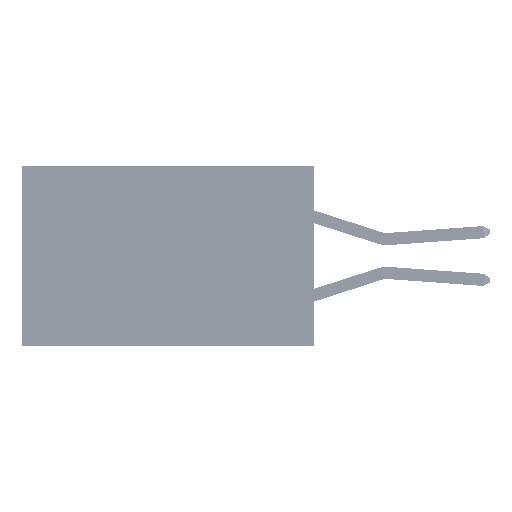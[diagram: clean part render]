
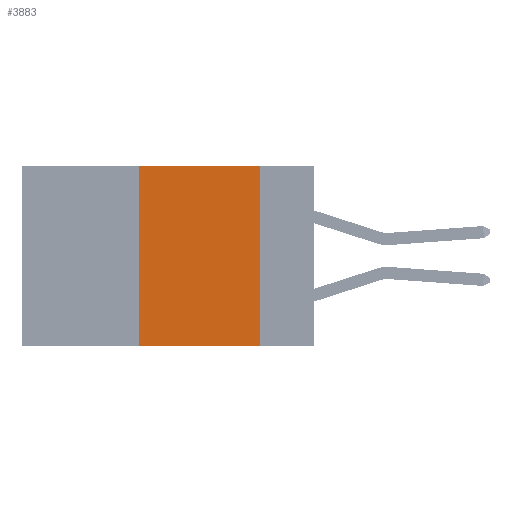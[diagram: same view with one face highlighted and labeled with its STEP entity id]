
A CAD part, left-side view. The second image highlights one B-rep face of the part: STEP entity #3883.
In plain terms, the highlighted planar face has unit normal (-1, 0, 0).
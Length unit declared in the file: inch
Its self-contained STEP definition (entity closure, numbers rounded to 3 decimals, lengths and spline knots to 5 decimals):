
#3260 = VERTEX_POINT ( 'NONE', #17033 ) ;
#3572 = AXIS2_PLACEMENT_3D ( 'NONE', #42598, #31420, #8607 ) ;
#3883 = ADVANCED_FACE ( 'NONE', ( #20816 ), #23751, .F. ) ;
#4056 = LINE ( 'NONE', #18762, #48701 ) ;
#6908 = DIRECTION ( 'NONE',  ( 0., -1., 0. ) ) ;
#8607 = DIRECTION ( 'NONE',  ( 0., 0., -1. ) ) ;
#8686 = DIRECTION ( 'NONE',  ( 0., 0., -1. ) ) ;
#10719 = EDGE_LOOP ( 'NONE', ( #48430, #15231, #14792, #28986 ) ) ;
#12511 = CARTESIAN_POINT ( 'NONE',  ( 0., 0.11, 0. ) ) ;
#13696 = CARTESIAN_POINT ( 'NONE',  ( 0., 0.11, -0.37 ) ) ;
#14792 = ORIENTED_EDGE ( 'NONE', *, *, #29529, .F. ) ;
#15231 = ORIENTED_EDGE ( 'NONE', *, *, #34833, .F. ) ;
#17016 = LINE ( 'NONE', #45388, #19379 ) ;
#17033 = CARTESIAN_POINT ( 'NONE',  ( 0., 0.11, 0. ) ) ;
#17497 = CARTESIAN_POINT ( 'NONE',  ( 0., 0.36, -0.37 ) ) ;
#18762 = CARTESIAN_POINT ( 'NONE',  ( 0., 0.6, 0. ) ) ;
#19090 = VECTOR ( 'NONE', #42324, 39.37008 ) ;
#19379 = VECTOR ( 'NONE', #46019, 39.37008 ) ;
#20316 = VERTEX_POINT ( 'NONE', #17497 ) ;
#20816 = FACE_OUTER_BOUND ( 'NONE', #10719, .T. ) ;
#21238 = CARTESIAN_POINT ( 'NONE',  ( 0., 0.36, 0. ) ) ;
#23751 = PLANE ( 'NONE',  #3572 ) ;
#25722 = VECTOR ( 'NONE', #8686, 39.37008 ) ;
#28986 = ORIENTED_EDGE ( 'NONE', *, *, #46115, .T. ) ;
#29529 = EDGE_CURVE ( 'NONE', #20316, #42090, #34529, .T. ) ;
#31420 = DIRECTION ( 'NONE',  ( 1., 0., 0. ) ) ;
#34529 = LINE ( 'NONE', #42477, #19090 ) ;
#34833 = EDGE_CURVE ( 'NONE', #42090, #3260, #4056, .T. ) ;
#40669 = EDGE_CURVE ( 'NONE', #3260, #48290, #45989, .T. ) ;
#42090 = VERTEX_POINT ( 'NONE', #21238 ) ;
#42324 = DIRECTION ( 'NONE',  ( 0., 0., 1. ) ) ;
#42477 = CARTESIAN_POINT ( 'NONE',  ( 0., 0.36, 0. ) ) ;
#42598 = CARTESIAN_POINT ( 'NONE',  ( 0., 0.6, 0. ) ) ;
#45388 = CARTESIAN_POINT ( 'NONE',  ( 0., 0.6, -0.37 ) ) ;
#45989 = LINE ( 'NONE', #12511, #25722 ) ;
#46019 = DIRECTION ( 'NONE',  ( 0., -1., 0. ) ) ;
#46115 = EDGE_CURVE ( 'NONE', #20316, #48290, #17016, .T. ) ;
#48290 = VERTEX_POINT ( 'NONE', #13696 ) ;
#48430 = ORIENTED_EDGE ( 'NONE', *, *, #40669, .F. ) ;
#48701 = VECTOR ( 'NONE', #6908, 39.37008 ) ;
